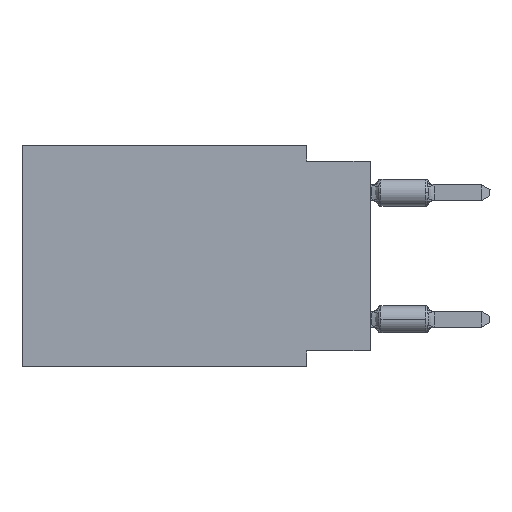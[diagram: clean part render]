
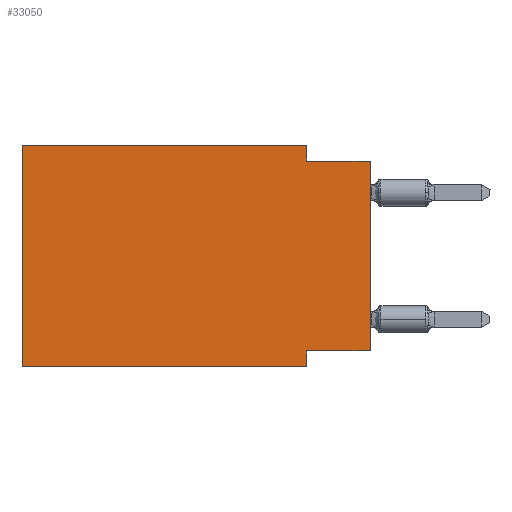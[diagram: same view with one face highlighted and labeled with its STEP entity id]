
A CAD part, left-side view. The second image highlights one B-rep face of the part: STEP entity #33050.
In plain terms, the highlighted planar face has unit normal (-1, 0, 0).
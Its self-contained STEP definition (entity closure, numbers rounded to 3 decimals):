
#217 = PLANE ( 'NONE',  #60472 ) ;
#531 = VECTOR ( 'NONE', #7813, 1000. ) ;
#1750 = CARTESIAN_POINT ( 'NONE',  ( 0., 0., -0.635 ) ) ;
#3804 = LINE ( 'NONE', #55634, #531 ) ;
#5718 = EDGE_LOOP ( 'NONE', ( #18444, #7103, #19247, #41480, #33348, #56353, #59858, #32324 ) ) ;
#5832 = LINE ( 'NONE', #24635, #51958 ) ;
#7103 = ORIENTED_EDGE ( 'NONE', *, *, #53252, .F. ) ;
#7813 = DIRECTION ( 'NONE',  ( 0., 0., 1. ) ) ;
#7965 = CARTESIAN_POINT ( 'NONE',  ( 0., 13.97, 0. ) ) ;
#8266 = DIRECTION ( 'NONE',  ( 0., -1., 0. ) ) ;
#9257 = CARTESIAN_POINT ( 'NONE',  ( 0., 13.97, 0. ) ) ;
#12606 = CARTESIAN_POINT ( 'NONE',  ( 0., 2.54, -8.89 ) ) ;
#12650 = VECTOR ( 'NONE', #20552, 1000. ) ;
#13290 = CARTESIAN_POINT ( 'NONE',  ( 0., 0., -0.635 ) ) ;
#16820 = VECTOR ( 'NONE', #43462, 1000. ) ;
#17667 = LINE ( 'NONE', #36490, #52993 ) ;
#18133 = LINE ( 'NONE', #7965, #57980 ) ;
#18444 = ORIENTED_EDGE ( 'NONE', *, *, #20771, .T. ) ;
#19247 = ORIENTED_EDGE ( 'NONE', *, *, #35196, .F. ) ;
#19549 = VERTEX_POINT ( 'NONE', #37195 ) ;
#20246 = LINE ( 'NONE', #1750, #12650 ) ;
#20552 = DIRECTION ( 'NONE',  ( 0., -1., 0. ) ) ;
#20771 = EDGE_CURVE ( 'NONE', #24783, #40896, #17667, .T. ) ;
#21587 = EDGE_CURVE ( 'NONE', #19549, #48882, #5832, .T. ) ;
#23836 = DIRECTION ( 'NONE',  ( 0., 1., 0. ) ) ;
#23938 = CARTESIAN_POINT ( 'NONE',  ( 0., 13.97, 0. ) ) ;
#24635 = CARTESIAN_POINT ( 'NONE',  ( 0., 13.97, -8.89 ) ) ;
#24783 = VERTEX_POINT ( 'NONE', #51501 ) ;
#25181 = CARTESIAN_POINT ( 'NONE',  ( 0., 2.54, -8.255 ) ) ;
#26921 = DIRECTION ( 'NONE',  ( 0., 0., 1. ) ) ;
#28468 = CARTESIAN_POINT ( 'NONE',  ( 0., 0., -8.255 ) ) ;
#28649 = EDGE_CURVE ( 'NONE', #52708, #48371, #18133, .T. ) ;
#31174 = CARTESIAN_POINT ( 'NONE',  ( 0., 2.54, 0. ) ) ;
#32324 = ORIENTED_EDGE ( 'NONE', *, *, #48076, .F. ) ;
#32756 = VERTEX_POINT ( 'NONE', #49884 ) ;
#33050 = ADVANCED_FACE ( 'NONE', ( #42165 ), #217, .F. ) ;
#33348 = ORIENTED_EDGE ( 'NONE', *, *, #46780, .F. ) ;
#35196 = EDGE_CURVE ( 'NONE', #48371, #32756, #41741, .T. ) ;
#36490 = CARTESIAN_POINT ( 'NONE',  ( 0., 0., 0. ) ) ;
#37195 = CARTESIAN_POINT ( 'NONE',  ( 0., 13.97, -8.89 ) ) ;
#37723 = DIRECTION ( 'NONE',  ( 0., 0., -1. ) ) ;
#37928 = CARTESIAN_POINT ( 'NONE',  ( 0., 2.54, -8.89 ) ) ;
#40896 = VERTEX_POINT ( 'NONE', #13290 ) ;
#41480 = ORIENTED_EDGE ( 'NONE', *, *, #28649, .F. ) ;
#41741 = LINE ( 'NONE', #47294, #43767 ) ;
#42165 = FACE_OUTER_BOUND ( 'NONE', #5718, .T. ) ;
#43462 = DIRECTION ( 'NONE',  ( 0., 0., -1. ) ) ;
#43481 = DIRECTION ( 'NONE',  ( 0., -1., 0. ) ) ;
#43767 = VECTOR ( 'NONE', #37723, 1000. ) ;
#46780 = EDGE_CURVE ( 'NONE', #19549, #52708, #3804, .T. ) ;
#47000 = LINE ( 'NONE', #28468, #51819 ) ;
#47294 = CARTESIAN_POINT ( 'NONE',  ( 0., 2.54, 0. ) ) ;
#47479 = LINE ( 'NONE', #37928, #16820 ) ;
#47802 = VERTEX_POINT ( 'NONE', #25181 ) ;
#48076 = EDGE_CURVE ( 'NONE', #24783, #47802, #47000, .T. ) ;
#48371 = VERTEX_POINT ( 'NONE', #31174 ) ;
#48882 = VERTEX_POINT ( 'NONE', #12606 ) ;
#49884 = CARTESIAN_POINT ( 'NONE',  ( 0., 2.54, -0.635 ) ) ;
#51501 = CARTESIAN_POINT ( 'NONE',  ( 0., 0., -8.255 ) ) ;
#51819 = VECTOR ( 'NONE', #23836, 1000. ) ;
#51958 = VECTOR ( 'NONE', #43481, 1000. ) ;
#52708 = VERTEX_POINT ( 'NONE', #9257 ) ;
#52993 = VECTOR ( 'NONE', #26921, 1000. ) ;
#53252 = EDGE_CURVE ( 'NONE', #32756, #40896, #20246, .T. ) ;
#55634 = CARTESIAN_POINT ( 'NONE',  ( 0., 13.97, 0. ) ) ;
#56353 = ORIENTED_EDGE ( 'NONE', *, *, #21587, .T. ) ;
#56670 = DIRECTION ( 'NONE',  ( 0., 0., -1. ) ) ;
#57980 = VECTOR ( 'NONE', #8266, 1000. ) ;
#58188 = EDGE_CURVE ( 'NONE', #47802, #48882, #47479, .T. ) ;
#59858 = ORIENTED_EDGE ( 'NONE', *, *, #58188, .F. ) ;
#60472 = AXIS2_PLACEMENT_3D ( 'NONE', #23938, #60978, #56670 ) ;
#60978 = DIRECTION ( 'NONE',  ( 1., 0., 0. ) ) ;
